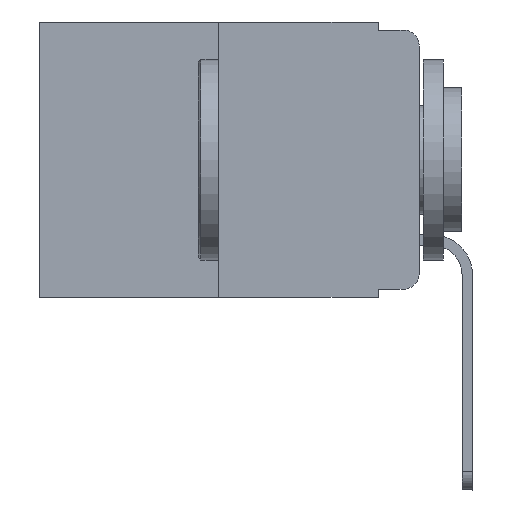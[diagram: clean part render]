
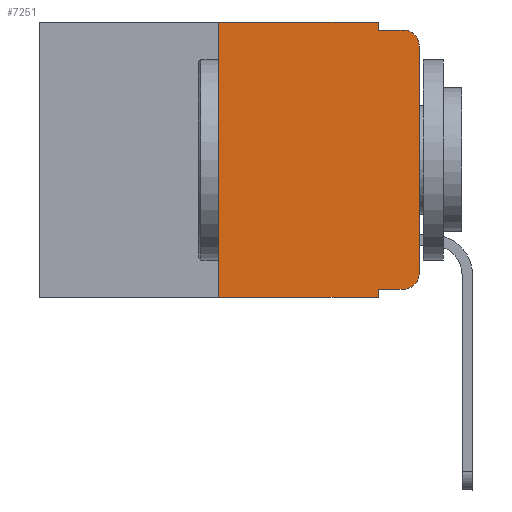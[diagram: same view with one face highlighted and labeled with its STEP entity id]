
A CAD part, left-side view. The second image highlights one B-rep face of the part: STEP entity #7251.
In plain terms, the highlighted planar face has unit normal (-1, 0, 0).
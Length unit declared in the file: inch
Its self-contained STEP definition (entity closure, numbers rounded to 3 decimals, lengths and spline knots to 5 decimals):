
#235 = DIRECTION ( 'NONE',  ( -1., 0., 0. ) ) ;
#788 = CARTESIAN_POINT ( 'NONE',  ( 0., 0.051, -0.333 ) ) ;
#888 = CARTESIAN_POINT ( 'NONE',  ( 0., 0.25, 0. ) ) ;
#1588 = CARTESIAN_POINT ( 'NONE',  ( 0., 0.051, -0.343 ) ) ;
#1733 = DIRECTION ( 'NONE',  ( 0., 0., -1. ) ) ;
#1914 = VECTOR ( 'NONE', #10859, 39.37008 ) ;
#2051 = EDGE_CURVE ( 'NONE', #14595, #22761, #17062, .T. ) ;
#2191 = ORIENTED_EDGE ( 'NONE', *, *, #22299, .F. ) ;
#2478 = CARTESIAN_POINT ( 'NONE',  ( 0., 0.051, 0. ) ) ;
#2588 = AXIS2_PLACEMENT_3D ( 'NONE', #18576, #18334, #22207 ) ;
#3003 = EDGE_CURVE ( 'NONE', #4212, #15186, #19632, .T. ) ;
#3023 = VECTOR ( 'NONE', #1733, 39.37008 ) ;
#3437 = VERTEX_POINT ( 'NONE', #19181 ) ;
#3439 = ORIENTED_EDGE ( 'NONE', *, *, #12883, .T. ) ;
#3974 = CARTESIAN_POINT ( 'NONE',  ( 0., 0.25, -0.343 ) ) ;
#4097 = LINE ( 'NONE', #15697, #21335 ) ;
#4212 = VERTEX_POINT ( 'NONE', #6779 ) ;
#4588 = CIRCLE ( 'NONE', #2588, 0.02 ) ;
#5359 = CARTESIAN_POINT ( 'NONE',  ( 0., 0.051, 0. ) ) ;
#5514 = LINE ( 'NONE', #13119, #1914 ) ;
#6279 = EDGE_LOOP ( 'NONE', ( #23434, #13510, #22404, #23065, #10474, #7051, #24671, #2191, #3439, #6413 ) ) ;
#6413 = ORIENTED_EDGE ( 'NONE', *, *, #3003, .T. ) ;
#6779 = CARTESIAN_POINT ( 'NONE',  ( 0., 0.02, -0.333 ) ) ;
#6889 = VERTEX_POINT ( 'NONE', #19011 ) ;
#6941 = DIRECTION ( 'NONE',  ( 0., 0., 1. ) ) ;
#6997 = VECTOR ( 'NONE', #16030, 39.37008 ) ;
#7051 = ORIENTED_EDGE ( 'NONE', *, *, #8897, .F. ) ;
#7103 = CARTESIAN_POINT ( 'NONE',  ( 0., 0., -0.313 ) ) ;
#7251 = ADVANCED_FACE ( 'NONE', ( #12990 ), #23566, .F. ) ;
#7443 = CARTESIAN_POINT ( 'NONE',  ( 0., 0.25, 0. ) ) ;
#7586 = AXIS2_PLACEMENT_3D ( 'NONE', #19802, #17452, #15949 ) ;
#8237 = DIRECTION ( 'NONE',  ( 0., 0., -1. ) ) ;
#8529 = LINE ( 'NONE', #788, #6997 ) ;
#8679 = VERTEX_POINT ( 'NONE', #2478 ) ;
#8897 = EDGE_CURVE ( 'NONE', #12279, #22164, #20664, .T. ) ;
#10429 = LINE ( 'NONE', #12552, #14600 ) ;
#10474 = ORIENTED_EDGE ( 'NONE', *, *, #16416, .F. ) ;
#10859 = DIRECTION ( 'NONE',  ( 0., -1., 0. ) ) ;
#12279 = VERTEX_POINT ( 'NONE', #3974 ) ;
#12487 = CARTESIAN_POINT ( 'NONE',  ( 0., 0.051, -0.01 ) ) ;
#12552 = CARTESIAN_POINT ( 'NONE',  ( 0., 0., 0. ) ) ;
#12883 = EDGE_CURVE ( 'NONE', #3437, #4212, #8529, .T. ) ;
#12990 = FACE_OUTER_BOUND ( 'NONE', #6279, .T. ) ;
#13119 = CARTESIAN_POINT ( 'NONE',  ( 0., 0.473, 0. ) ) ;
#13367 = EDGE_CURVE ( 'NONE', #8679, #14595, #15210, .T. ) ;
#13444 = VECTOR ( 'NONE', #15119, 39.37008 ) ;
#13510 = ORIENTED_EDGE ( 'NONE', *, *, #19689, .T. ) ;
#13616 = VECTOR ( 'NONE', #24560, 39.37008 ) ;
#13671 = EDGE_CURVE ( 'NONE', #15186, #6889, #10429, .T. ) ;
#13688 = DIRECTION ( 'NONE',  ( 0., -1., 0. ) ) ;
#13991 = VECTOR ( 'NONE', #20909, 39.37008 ) ;
#14595 = VERTEX_POINT ( 'NONE', #12487 ) ;
#14600 = VECTOR ( 'NONE', #6941, 39.37008 ) ;
#15119 = DIRECTION ( 'NONE',  ( 0., 0., -1. ) ) ;
#15186 = VERTEX_POINT ( 'NONE', #7103 ) ;
#15210 = LINE ( 'NONE', #5359, #3023 ) ;
#15697 = CARTESIAN_POINT ( 'NONE',  ( 0., 0.473, -0.343 ) ) ;
#15949 = DIRECTION ( 'NONE',  ( 0., 0., -1. ) ) ;
#16030 = DIRECTION ( 'NONE',  ( 0., -1., 0. ) ) ;
#16416 = EDGE_CURVE ( 'NONE', #22164, #8679, #5514, .T. ) ;
#16877 = LINE ( 'NONE', #22870, #13444 ) ;
#17062 = LINE ( 'NONE', #24682, #13991 ) ;
#17452 = DIRECTION ( 'NONE',  ( 1., 0., 0. ) ) ;
#18334 = DIRECTION ( 'NONE',  ( -1., 0., 0. ) ) ;
#18576 = CARTESIAN_POINT ( 'NONE',  ( 0., 0.02, -0.03 ) ) ;
#19011 = CARTESIAN_POINT ( 'NONE',  ( 0., 0., -0.03 ) ) ;
#19181 = CARTESIAN_POINT ( 'NONE',  ( 0., 0.051, -0.333 ) ) ;
#19632 = CIRCLE ( 'NONE', #22852, 0.02 ) ;
#19689 = EDGE_CURVE ( 'NONE', #6889, #22761, #4588, .T. ) ;
#19802 = CARTESIAN_POINT ( 'NONE',  ( 0., 0.473, 0. ) ) ;
#19891 = EDGE_CURVE ( 'NONE', #12279, #21419, #4097, .T. ) ;
#20664 = LINE ( 'NONE', #7443, #13616 ) ;
#20830 = CARTESIAN_POINT ( 'NONE',  ( 0., 0.02, -0.01 ) ) ;
#20909 = DIRECTION ( 'NONE',  ( 0., -1., 0. ) ) ;
#21335 = VECTOR ( 'NONE', #13688, 39.37008 ) ;
#21419 = VERTEX_POINT ( 'NONE', #1588 ) ;
#22164 = VERTEX_POINT ( 'NONE', #888 ) ;
#22207 = DIRECTION ( 'NONE',  ( 0., 0., -1. ) ) ;
#22299 = EDGE_CURVE ( 'NONE', #3437, #21419, #16877, .T. ) ;
#22404 = ORIENTED_EDGE ( 'NONE', *, *, #2051, .F. ) ;
#22761 = VERTEX_POINT ( 'NONE', #20830 ) ;
#22852 = AXIS2_PLACEMENT_3D ( 'NONE', #23215, #235, #8237 ) ;
#22870 = CARTESIAN_POINT ( 'NONE',  ( 0., 0.051, 0. ) ) ;
#23065 = ORIENTED_EDGE ( 'NONE', *, *, #13367, .F. ) ;
#23215 = CARTESIAN_POINT ( 'NONE',  ( 0., 0.02, -0.313 ) ) ;
#23434 = ORIENTED_EDGE ( 'NONE', *, *, #13671, .T. ) ;
#23566 = PLANE ( 'NONE',  #7586 ) ;
#24560 = DIRECTION ( 'NONE',  ( 0., 0., 1. ) ) ;
#24671 = ORIENTED_EDGE ( 'NONE', *, *, #19891, .T. ) ;
#24682 = CARTESIAN_POINT ( 'NONE',  ( 0., 0.051, -0.01 ) ) ;
